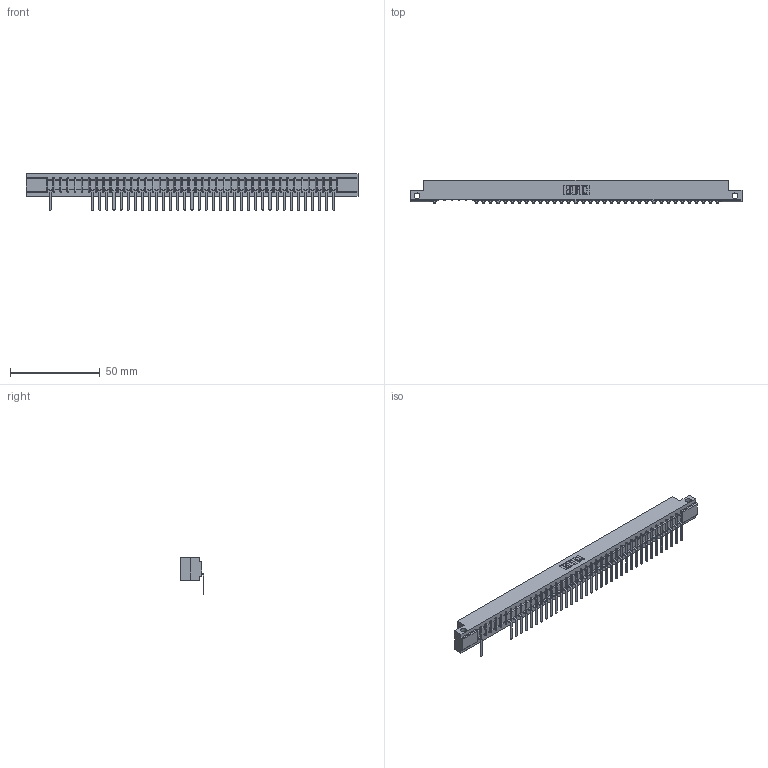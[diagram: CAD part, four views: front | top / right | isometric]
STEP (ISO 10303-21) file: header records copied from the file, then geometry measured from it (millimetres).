
FILE_DESCRIPTION (( 'STEP AP203' ), '1' );
FILE_NAME ('357-041-557-112.STEP', '2018-08-11T07:27:02', ( '' ), ( '' ), 'SwSTEP 2.0', 'SolidWorks 2016', '' );
FILE_SCHEMA (( 'CONFIG_CONTROL_DESIGN' ));
Length unit declared in the file: inch
Products named in the file (3): 307 Part_.128 Dia Side Mounting Holes; 307-290-002_557; 357-041-557-112
Assembly tree (37 placements, depth 2):
  357-041-557-112
    307 Part_.128 Dia Side Mounting Holes
    307-290-002_557  x36
Bounding box: 185.47 x 13.32 x 20.66 mm (x, y, z)
Volume: 19650.6 mm3; surface area: 24379.7 mm2
Topology: 37 solids, 37 shells, 3068 faces, 9427 edges, 6170 vertices
Faces by surface type: plane 1822, cylinder 1162, sphere 84
Entity records: 35968 total; most frequent: CARTESIAN_POINT 6091, ORIENTED_EDGE 6086, DIRECTION 5913, EDGE_CURVE 3043, VECTOR 2329, LINE 2329, VERTEX_POINT 1970, AXIS2_PLACEMENT_3D 1792
